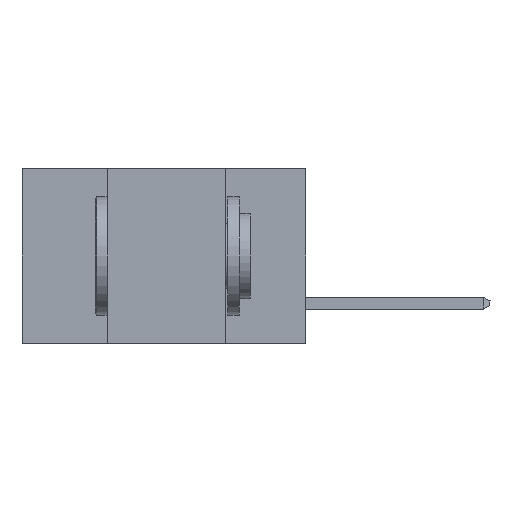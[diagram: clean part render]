
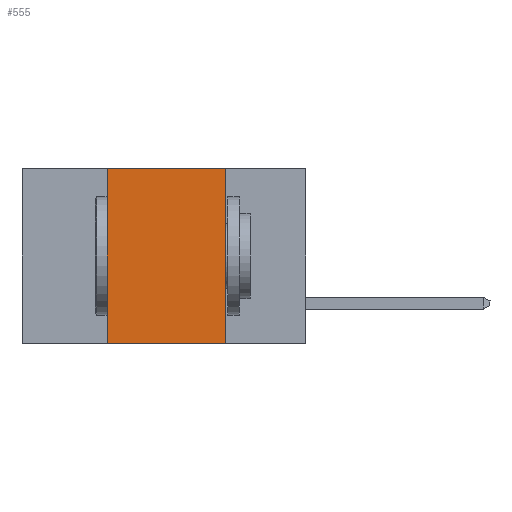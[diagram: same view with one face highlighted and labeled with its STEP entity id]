
A CAD part, left-side view. The second image highlights one B-rep face of the part: STEP entity #555.
In plain terms, the highlighted planar face has unit normal (-1, 0, 0).
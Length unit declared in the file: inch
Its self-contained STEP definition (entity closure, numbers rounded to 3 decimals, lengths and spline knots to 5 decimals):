
#212 = VECTOR ( 'NONE', #5806, 39.37008 ) ;
#555 = ADVANCED_FACE ( 'NONE', ( #12785 ), #1574, .F. ) ;
#1515 = EDGE_LOOP ( 'NONE', ( #3785, #5335, #1661, #16394 ) ) ;
#1574 = PLANE ( 'NONE',  #9471 ) ;
#1661 = ORIENTED_EDGE ( 'NONE', *, *, #9398, .F. ) ;
#2147 = DIRECTION ( 'NONE',  ( 0., 0., 1. ) ) ;
#2561 = LINE ( 'NONE', #6970, #212 ) ;
#3240 = DIRECTION ( 'NONE',  ( 1., 0., 0. ) ) ;
#3313 = LINE ( 'NONE', #17775, #6659 ) ;
#3647 = CARTESIAN_POINT ( 'NONE',  ( 0., 0.6, 0. ) ) ;
#3785 = ORIENTED_EDGE ( 'NONE', *, *, #7176, .F. ) ;
#4790 = VERTEX_POINT ( 'NONE', #19655 ) ;
#4872 = DIRECTION ( 'NONE',  ( 0., 0., -1. ) ) ;
#4902 = DIRECTION ( 'NONE',  ( 0., 0., -1. ) ) ;
#5335 = ORIENTED_EDGE ( 'NONE', *, *, #18761, .F. ) ;
#5806 = DIRECTION ( 'NONE',  ( 0., -1., 0. ) ) ;
#6659 = VECTOR ( 'NONE', #4872, 39.37008 ) ;
#6970 = CARTESIAN_POINT ( 'NONE',  ( 0., 0.6, -0.37 ) ) ;
#7176 = EDGE_CURVE ( 'NONE', #4790, #12632, #3313, .T. ) ;
#8457 = DIRECTION ( 'NONE',  ( 0., -1., 0. ) ) ;
#9398 = EDGE_CURVE ( 'NONE', #13005, #19154, #11696, .T. ) ;
#9471 = AXIS2_PLACEMENT_3D ( 'NONE', #3647, #3240, #4902 ) ;
#11696 = LINE ( 'NONE', #16511, #15007 ) ;
#12632 = VERTEX_POINT ( 'NONE', #19177 ) ;
#12785 = FACE_OUTER_BOUND ( 'NONE', #1515, .T. ) ;
#13005 = VERTEX_POINT ( 'NONE', #14057 ) ;
#14057 = CARTESIAN_POINT ( 'NONE',  ( 0., 0.42, -0.37 ) ) ;
#14881 = LINE ( 'NONE', #19682, #16269 ) ;
#15007 = VECTOR ( 'NONE', #2147, 39.37008 ) ;
#16269 = VECTOR ( 'NONE', #8457, 39.37008 ) ;
#16394 = ORIENTED_EDGE ( 'NONE', *, *, #19258, .T. ) ;
#16511 = CARTESIAN_POINT ( 'NONE',  ( 0., 0.42, -0.37 ) ) ;
#17775 = CARTESIAN_POINT ( 'NONE',  ( 0., 0.17, -0.37 ) ) ;
#17873 = CARTESIAN_POINT ( 'NONE',  ( 0., 0.42, 0. ) ) ;
#18761 = EDGE_CURVE ( 'NONE', #19154, #4790, #14881, .T. ) ;
#19154 = VERTEX_POINT ( 'NONE', #17873 ) ;
#19177 = CARTESIAN_POINT ( 'NONE',  ( 0., 0.17, -0.37 ) ) ;
#19258 = EDGE_CURVE ( 'NONE', #13005, #12632, #2561, .T. ) ;
#19655 = CARTESIAN_POINT ( 'NONE',  ( 0., 0.17, 0. ) ) ;
#19682 = CARTESIAN_POINT ( 'NONE',  ( 0., 0.6, 0. ) ) ;
